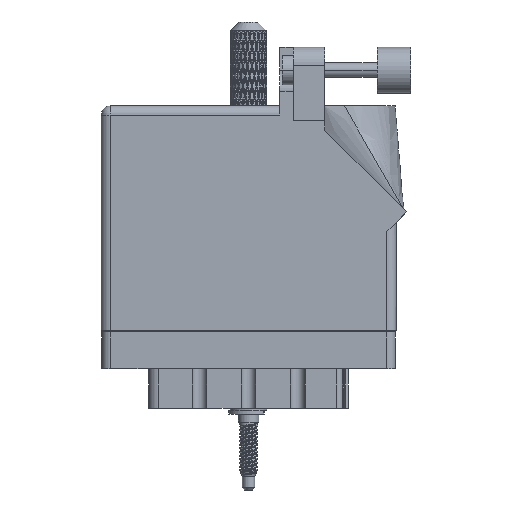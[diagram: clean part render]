
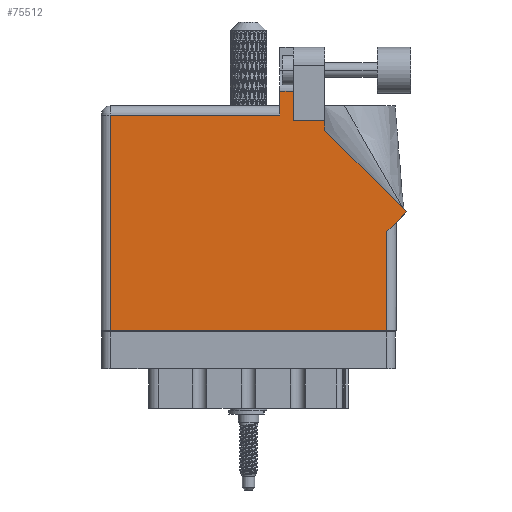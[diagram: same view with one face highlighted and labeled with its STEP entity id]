
A CAD part, front view. The second image highlights one B-rep face of the part: STEP entity #75512.
In plain terms, the highlighted face is planar.
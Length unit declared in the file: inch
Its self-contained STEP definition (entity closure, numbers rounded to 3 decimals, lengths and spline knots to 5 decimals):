
#1506 = VERTEX_POINT ( 'NONE', #82425 ) ;
#4037 = LINE ( 'NONE', #101256, #58467 ) ;
#5433 = VECTOR ( 'NONE', #86702, 39.37008 ) ;
#6942 = CARTESIAN_POINT ( 'NONE',  ( 0.062, 1.468, 0. ) ) ;
#7592 = ORIENTED_EDGE ( 'NONE', *, *, #50245, .T. ) ;
#7959 = VECTOR ( 'NONE', #29521, 39.37008 ) ;
#8521 = ORIENTED_EDGE ( 'NONE', *, *, #78171, .T. ) ;
#8683 = DIRECTION ( 'NONE',  ( -1., 0., 0. ) ) ;
#9842 = CARTESIAN_POINT ( 'NONE',  ( 0.062, 0., 0. ) ) ;
#10955 = VERTEX_POINT ( 'NONE', #79102 ) ;
#11618 = ORIENTED_EDGE ( 'NONE', *, *, #29424, .T. ) ;
#12716 = VECTOR ( 'NONE', #52537, 39.37008 ) ;
#15783 = LINE ( 'NONE', #103000, #5433 ) ;
#16334 = EDGE_CURVE ( 'NONE', #90462, #36146, #20677, .T. ) ;
#16672 = EDGE_CURVE ( 'NONE', #106663, #1506, #15783, .T. ) ;
#18090 = CARTESIAN_POINT ( 'NONE',  ( 1.524, 1.36442, 0. ) ) ;
#18158 = CARTESIAN_POINT ( 'NONE',  ( 1.524, 1.43, 0. ) ) ;
#20677 = LINE ( 'NONE', #105616, #77669 ) ;
#20886 = LINE ( 'NONE', #55343, #24843 ) ;
#21067 = CARTESIAN_POINT ( 'NONE',  ( 1.524, 1.43, 0. ) ) ;
#24542 = VECTOR ( 'NONE', #92309, 39.37008 ) ;
#24843 = VECTOR ( 'NONE', #80720, 39.37008 ) ;
#25944 = ORIENTED_EDGE ( 'NONE', *, *, #26845, .T. ) ;
#26845 = EDGE_CURVE ( 'NONE', #68538, #10955, #87095, .T. ) ;
#27860 = LINE ( 'NONE', #98597, #66726 ) ;
#28892 = FACE_OUTER_BOUND ( 'NONE', #39969, .T. ) ;
#29424 = EDGE_CURVE ( 'NONE', #66081, #38792, #27860, .T. ) ;
#29521 = DIRECTION ( 'NONE',  ( -0.707, 0.707, 0. ) ) ;
#32211 = LINE ( 'NONE', #18158, #12716 ) ;
#32679 = EDGE_CURVE ( 'NONE', #100796, #68538, #20886, .T. ) ;
#33046 = CARTESIAN_POINT ( 'NONE',  ( 1.217, 1.6315, 0. ) ) ;
#33136 = EDGE_CURVE ( 'NONE', #1506, #90462, #77881, .T. ) ;
#36146 = VERTEX_POINT ( 'NONE', #21067 ) ;
#37739 = AXIS2_PLACEMENT_3D ( 'NONE', #41138, #74439, #51937 ) ;
#38792 = VERTEX_POINT ( 'NONE', #55424 ) ;
#39430 = CARTESIAN_POINT ( 'NONE',  ( 1.64177, 1.6315, 0. ) ) ;
#39969 = EDGE_LOOP ( 'NONE', ( #40350, #66625, #11618, #7592, #96204, #25944, #8521, #71184, #41647, #52464, #104416 ) ) ;
#40350 = ORIENTED_EDGE ( 'NONE', *, *, #61580, .T. ) ;
#41138 = CARTESIAN_POINT ( 'NONE',  ( 0., 1.53, 0. ) ) ;
#41647 = ORIENTED_EDGE ( 'NONE', *, *, #33136, .T. ) ;
#42925 = CARTESIAN_POINT ( 'NONE',  ( 1.948, 0.675, 0. ) ) ;
#45839 = VECTOR ( 'NONE', #56766, 39.37008 ) ;
#49034 = VECTOR ( 'NONE', #8683, 39.37008 ) ;
#50245 = EDGE_CURVE ( 'NONE', #38792, #100796, #71068, .T. ) ;
#50555 = DIRECTION ( 'NONE',  ( 0., 1., 0. ) ) ;
#51937 = DIRECTION ( 'NONE',  ( -1., 0., 0. ) ) ;
#52464 = ORIENTED_EDGE ( 'NONE', *, *, #16334, .T. ) ;
#52537 = DIRECTION ( 'NONE',  ( -1., 0., 0. ) ) ;
#55343 = CARTESIAN_POINT ( 'NONE',  ( 0.062, 0., 0. ) ) ;
#55424 = CARTESIAN_POINT ( 'NONE',  ( 1.217, 1.468, 0. ) ) ;
#56200 = EDGE_CURVE ( 'NONE', #60381, #66081, #65252, .T. ) ;
#56766 = DIRECTION ( 'NONE',  ( -1., 0., 0. ) ) ;
#58467 = VECTOR ( 'NONE', #50555, 39.37008 ) ;
#60381 = VERTEX_POINT ( 'NONE', #97282 ) ;
#61580 = EDGE_CURVE ( 'NONE', #91049, #60381, #4037, .T. ) ;
#65252 = LINE ( 'NONE', #39430, #45839 ) ;
#66081 = VERTEX_POINT ( 'NONE', #33046 ) ;
#66625 = ORIENTED_EDGE ( 'NONE', *, *, #56200, .T. ) ;
#66726 = VECTOR ( 'NONE', #94226, 39.37008 ) ;
#66809 = PLANE ( 'NONE',  #37739 ) ;
#68538 = VERTEX_POINT ( 'NONE', #9842 ) ;
#70617 = CARTESIAN_POINT ( 'NONE',  ( 0., 0., 0. ) ) ;
#71068 = LINE ( 'NONE', #82941, #49034 ) ;
#71152 = CARTESIAN_POINT ( 'NONE',  ( 1.311, 1.43, 0. ) ) ;
#71184 = ORIENTED_EDGE ( 'NONE', *, *, #16672, .T. ) ;
#73822 = LINE ( 'NONE', #77019, #24542 ) ;
#74439 = DIRECTION ( 'NONE',  ( 0., 0., -1. ) ) ;
#75512 = ADVANCED_FACE ( 'NONE', ( #28892 ), #66809, .F. ) ;
#77019 = CARTESIAN_POINT ( 'NONE',  ( 1.948, 0.737, 0. ) ) ;
#77669 = VECTOR ( 'NONE', #97310, 39.37008 ) ;
#77881 = LINE ( 'NONE', #86777, #7959 ) ;
#78171 = EDGE_CURVE ( 'NONE', #10955, #106663, #73822, .T. ) ;
#79102 = CARTESIAN_POINT ( 'NONE',  ( 1.948, 0., 0. ) ) ;
#80720 = DIRECTION ( 'NONE',  ( 0., -1., 0. ) ) ;
#82425 = CARTESIAN_POINT ( 'NONE',  ( 2.08071, 0.80771, 0. ) ) ;
#82941 = CARTESIAN_POINT ( 'NONE',  ( 0., 1.468, 0. ) ) ;
#83916 = EDGE_CURVE ( 'NONE', #36146, #91049, #32211, .T. ) ;
#86702 = DIRECTION ( 'NONE',  ( 0.707, 0.707, 0. ) ) ;
#86777 = CARTESIAN_POINT ( 'NONE',  ( 2.08071, 0.80771, 0. ) ) ;
#87095 = LINE ( 'NONE', #70617, #97503 ) ;
#90462 = VERTEX_POINT ( 'NONE', #18090 ) ;
#91049 = VERTEX_POINT ( 'NONE', #71152 ) ;
#92309 = DIRECTION ( 'NONE',  ( 0., 1., 0. ) ) ;
#94226 = DIRECTION ( 'NONE',  ( 0., -1., 0. ) ) ;
#96204 = ORIENTED_EDGE ( 'NONE', *, *, #32679, .T. ) ;
#97282 = CARTESIAN_POINT ( 'NONE',  ( 1.311, 1.6315, 0. ) ) ;
#97310 = DIRECTION ( 'NONE',  ( 0., 1., 0. ) ) ;
#97503 = VECTOR ( 'NONE', #106140, 39.37008 ) ;
#98597 = CARTESIAN_POINT ( 'NONE',  ( 1.217, 1.53, 0. ) ) ;
#100796 = VERTEX_POINT ( 'NONE', #6942 ) ;
#101256 = CARTESIAN_POINT ( 'NONE',  ( 1.311, 1.43, 0. ) ) ;
#103000 = CARTESIAN_POINT ( 'NONE',  ( 2.01, 0.737, 0. ) ) ;
#104416 = ORIENTED_EDGE ( 'NONE', *, *, #83916, .T. ) ;
#105616 = CARTESIAN_POINT ( 'NONE',  ( 1.524, 1.36442, 0. ) ) ;
#106140 = DIRECTION ( 'NONE',  ( 1., 0., 0. ) ) ;
#106663 = VERTEX_POINT ( 'NONE', #42925 ) ;
